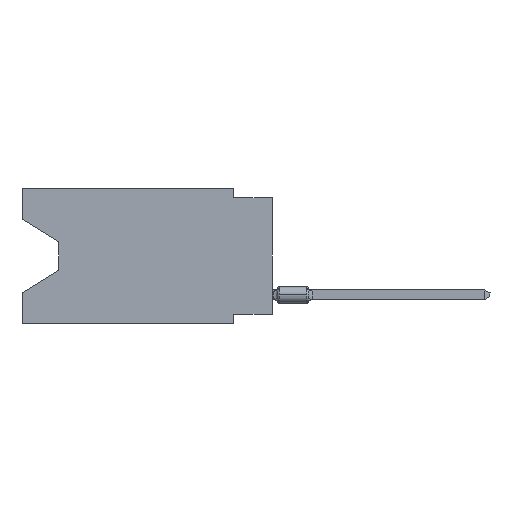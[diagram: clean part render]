
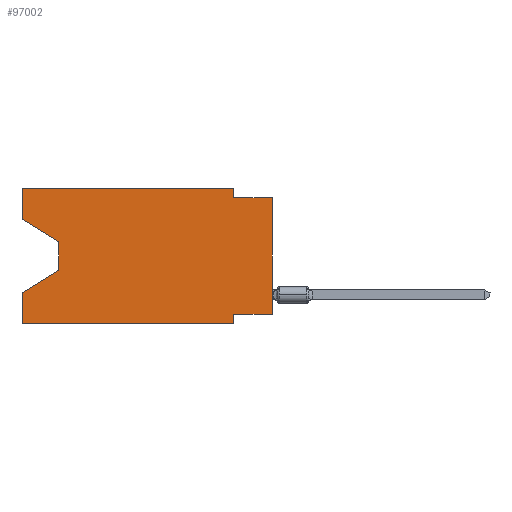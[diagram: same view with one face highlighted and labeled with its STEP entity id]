
A CAD part, left-side view. The second image highlights one B-rep face of the part: STEP entity #97002.
In plain terms, the highlighted planar face has unit normal (-1, 0, 0).
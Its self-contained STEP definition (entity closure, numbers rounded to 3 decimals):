
#1265 = DIRECTION ( 'NONE',  ( 0., -1., 0. ) ) ;
#1271 = CARTESIAN_POINT ( 'NONE',  ( 0., 2.54, -8.89 ) ) ;
#1537 = VECTOR ( 'NONE', #29214, 1000. ) ;
#1701 = VERTEX_POINT ( 'NONE', #84476 ) ;
#2234 = VERTEX_POINT ( 'NONE', #94891 ) ;
#4462 = VECTOR ( 'NONE', #29680, 1000. ) ;
#4634 = VERTEX_POINT ( 'NONE', #73875 ) ;
#5273 = CARTESIAN_POINT ( 'NONE',  ( 0., 16.383, -8.89 ) ) ;
#6755 = CARTESIAN_POINT ( 'NONE',  ( 0., 16.383, 0. ) ) ;
#7004 = CARTESIAN_POINT ( 'NONE',  ( 0., 16.383, -6.852 ) ) ;
#7314 = LINE ( 'NONE', #41348, #106340 ) ;
#7990 = CARTESIAN_POINT ( 'NONE',  ( 0., 2.54, -0.635 ) ) ;
#8046 = EDGE_CURVE ( 'NONE', #78390, #71857, #13650, .T. ) ;
#8804 = VECTOR ( 'NONE', #10252, 1000. ) ;
#10252 = DIRECTION ( 'NONE',  ( 0., 1., 0. ) ) ;
#13650 = LINE ( 'NONE', #5273, #81510 ) ;
#14146 = CARTESIAN_POINT ( 'NONE',  ( 0., 2.54, -8.255 ) ) ;
#15672 = DIRECTION ( 'NONE',  ( 0., 0., -1. ) ) ;
#16218 = CARTESIAN_POINT ( 'NONE',  ( 0., 13.97, -3.505 ) ) ;
#16574 = ORIENTED_EDGE ( 'NONE', *, *, #71065, .T. ) ;
#17334 = DIRECTION ( 'NONE',  ( 0., 0., 1. ) ) ;
#18227 = ORIENTED_EDGE ( 'NONE', *, *, #87553, .F. ) ;
#18282 = CARTESIAN_POINT ( 'NONE',  ( 0., 0., -0.635 ) ) ;
#18567 = LINE ( 'NONE', #35304, #27028 ) ;
#19297 = LINE ( 'NONE', #44967, #69276 ) ;
#21711 = DIRECTION ( 'NONE',  ( 0., 0., 1. ) ) ;
#22188 = EDGE_CURVE ( 'NONE', #44675, #86809, #50707, .T. ) ;
#26701 = CARTESIAN_POINT ( 'NONE',  ( 0., 16.383, -2.038 ) ) ;
#26828 = EDGE_CURVE ( 'NONE', #1701, #40441, #18567, .T. ) ;
#27028 = VECTOR ( 'NONE', #1265, 1000. ) ;
#27382 = ORIENTED_EDGE ( 'NONE', *, *, #47919, .T. ) ;
#29212 = ORIENTED_EDGE ( 'NONE', *, *, #63512, .F. ) ;
#29214 = DIRECTION ( 'NONE',  ( 0., 0., 1. ) ) ;
#29680 = DIRECTION ( 'NONE',  ( 0., -0.855, -0.519 ) ) ;
#29894 = ORIENTED_EDGE ( 'NONE', *, *, #22188, .F. ) ;
#31036 = ORIENTED_EDGE ( 'NONE', *, *, #89635, .F. ) ;
#33798 = EDGE_CURVE ( 'NONE', #39761, #4634, #34386, .T. ) ;
#33980 = CARTESIAN_POINT ( 'NONE',  ( 0., 0., -0.635 ) ) ;
#34386 = LINE ( 'NONE', #101850, #59392 ) ;
#35304 = CARTESIAN_POINT ( 'NONE',  ( 0., 16.383, 0. ) ) ;
#36595 = DIRECTION ( 'NONE',  ( 0., 0., -1. ) ) ;
#36893 = VECTOR ( 'NONE', #17334, 1000. ) ;
#37671 = DIRECTION ( 'NONE',  ( 0., -1., 0. ) ) ;
#39123 = ORIENTED_EDGE ( 'NONE', *, *, #33798, .T. ) ;
#39761 = VERTEX_POINT ( 'NONE', #16218 ) ;
#40441 = VERTEX_POINT ( 'NONE', #61227 ) ;
#40783 = DIRECTION ( 'NONE',  ( 1., 0., 0. ) ) ;
#41348 = CARTESIAN_POINT ( 'NONE',  ( 0., 2.54, -8.89 ) ) ;
#41872 = VERTEX_POINT ( 'NONE', #7004 ) ;
#43462 = CARTESIAN_POINT ( 'NONE',  ( 0., 16.383, -8.89 ) ) ;
#44675 = VERTEX_POINT ( 'NONE', #7990 ) ;
#44967 = CARTESIAN_POINT ( 'NONE',  ( 0., 2.54, 0. ) ) ;
#47919 = EDGE_CURVE ( 'NONE', #101763, #39761, #89879, .T. ) ;
#48395 = EDGE_CURVE ( 'NONE', #2234, #86809, #79753, .T. ) ;
#50707 = LINE ( 'NONE', #33980, #100738 ) ;
#51547 = CARTESIAN_POINT ( 'NONE',  ( 0., 0., -8.255 ) ) ;
#54509 = CARTESIAN_POINT ( 'NONE',  ( 0., 13.97, -5.385 ) ) ;
#55303 = CARTESIAN_POINT ( 'NONE',  ( 0., 16.383, -2.038 ) ) ;
#56640 = VERTEX_POINT ( 'NONE', #14146 ) ;
#57534 = FACE_OUTER_BOUND ( 'NONE', #86968, .T. ) ;
#58635 = LINE ( 'NONE', #74825, #36893 ) ;
#59392 = VECTOR ( 'NONE', #68394, 1000. ) ;
#61227 = CARTESIAN_POINT ( 'NONE',  ( 0., 2.54, 0. ) ) ;
#63402 = LINE ( 'NONE', #54509, #98955 ) ;
#63512 = EDGE_CURVE ( 'NONE', #101763, #1701, #63746, .T. ) ;
#63746 = LINE ( 'NONE', #71024, #1537 ) ;
#64065 = CARTESIAN_POINT ( 'NONE',  ( 0., 0., 0. ) ) ;
#68005 = DIRECTION ( 'NONE',  ( 0., -1., 0. ) ) ;
#68391 = ORIENTED_EDGE ( 'NONE', *, *, #8046, .T. ) ;
#68394 = DIRECTION ( 'NONE',  ( 0., 0., -1. ) ) ;
#69276 = VECTOR ( 'NONE', #36595, 1000. ) ;
#71024 = CARTESIAN_POINT ( 'NONE',  ( 0., 16.383, 0. ) ) ;
#71065 = EDGE_CURVE ( 'NONE', #4634, #41872, #63402, .T. ) ;
#71857 = VERTEX_POINT ( 'NONE', #1271 ) ;
#72581 = ORIENTED_EDGE ( 'NONE', *, *, #87468, .F. ) ;
#73875 = CARTESIAN_POINT ( 'NONE',  ( 0., 13.97, -5.385 ) ) ;
#74825 = CARTESIAN_POINT ( 'NONE',  ( 0., 16.383, 0. ) ) ;
#76754 = AXIS2_PLACEMENT_3D ( 'NONE', #6755, #40783, #15672 ) ;
#77584 = EDGE_CURVE ( 'NONE', #2234, #56640, #102280, .T. ) ;
#78390 = VERTEX_POINT ( 'NONE', #43462 ) ;
#79753 = LINE ( 'NONE', #64065, #107860 ) ;
#79937 = ORIENTED_EDGE ( 'NONE', *, *, #26828, .F. ) ;
#81510 = VECTOR ( 'NONE', #37671, 1000. ) ;
#84476 = CARTESIAN_POINT ( 'NONE',  ( 0., 16.383, 0. ) ) ;
#86809 = VERTEX_POINT ( 'NONE', #18282 ) ;
#86968 = EDGE_LOOP ( 'NONE', ( #27382, #39123, #16574, #72581, #68391, #18227, #91033, #94903, #29894, #31036, #79937, #29212 ) ) ;
#87468 = EDGE_CURVE ( 'NONE', #78390, #41872, #58635, .T. ) ;
#87553 = EDGE_CURVE ( 'NONE', #56640, #71857, #7314, .T. ) ;
#89635 = EDGE_CURVE ( 'NONE', #40441, #44675, #19297, .T. ) ;
#89879 = LINE ( 'NONE', #55303, #4462 ) ;
#91033 = ORIENTED_EDGE ( 'NONE', *, *, #77584, .F. ) ;
#91543 = PLANE ( 'NONE',  #76754 ) ;
#94891 = CARTESIAN_POINT ( 'NONE',  ( 0., 0., -8.255 ) ) ;
#94903 = ORIENTED_EDGE ( 'NONE', *, *, #48395, .T. ) ;
#96337 = DIRECTION ( 'NONE',  ( 0., 0.855, -0.519 ) ) ;
#97002 = ADVANCED_FACE ( 'NONE', ( #57534 ), #91543, .F. ) ;
#98955 = VECTOR ( 'NONE', #96337, 1000. ) ;
#100738 = VECTOR ( 'NONE', #68005, 1000. ) ;
#101763 = VERTEX_POINT ( 'NONE', #26701 ) ;
#101850 = CARTESIAN_POINT ( 'NONE',  ( 0., 13.97, -3.505 ) ) ;
#102280 = LINE ( 'NONE', #51547, #8804 ) ;
#106340 = VECTOR ( 'NONE', #109348, 1000. ) ;
#107860 = VECTOR ( 'NONE', #21711, 1000. ) ;
#109348 = DIRECTION ( 'NONE',  ( 0., 0., -1. ) ) ;
